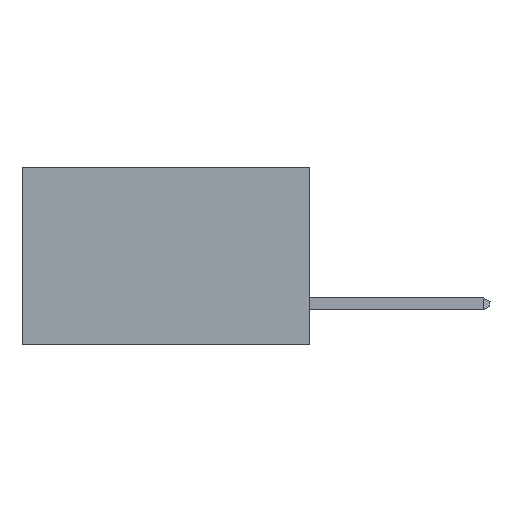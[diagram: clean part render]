
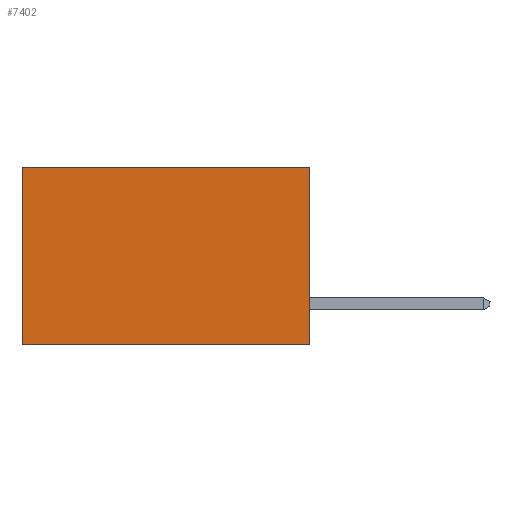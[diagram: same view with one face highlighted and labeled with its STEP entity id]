
A CAD part, left-side view. The second image highlights one B-rep face of the part: STEP entity #7402.
In plain terms, the highlighted planar face has unit normal (-1, 0, 0).
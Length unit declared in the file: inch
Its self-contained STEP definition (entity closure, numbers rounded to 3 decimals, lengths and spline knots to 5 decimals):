
#2269 = VECTOR ( 'NONE', #13233, 39.37008 ) ;
#2680 = LINE ( 'NONE', #18093, #2269 ) ;
#3606 = ORIENTED_EDGE ( 'NONE', *, *, #5074, .F. ) ;
#5074 = EDGE_CURVE ( 'NONE', #19705, #22092, #2680, .T. ) ;
#6584 = EDGE_CURVE ( 'NONE', #19705, #29613, #7545, .T. ) ;
#7337 = DIRECTION ( 'NONE',  ( 0., 0., -1. ) ) ;
#7402 = ADVANCED_FACE ( 'NONE', ( #11373 ), #29030, .F. ) ;
#7545 = LINE ( 'NONE', #10958, #28023 ) ;
#8301 = ORIENTED_EDGE ( 'NONE', *, *, #22850, .T. ) ;
#8864 = LINE ( 'NONE', #15539, #23919 ) ;
#9128 = ORIENTED_EDGE ( 'NONE', *, *, #9698, .F. ) ;
#9698 = EDGE_CURVE ( 'NONE', #22092, #19386, #8864, .T. ) ;
#10958 = CARTESIAN_POINT ( 'NONE',  ( 0.2875, 0., 0. ) ) ;
#11373 = FACE_OUTER_BOUND ( 'NONE', #11970, .T. ) ;
#11970 = EDGE_LOOP ( 'NONE', ( #8301, #9128, #3606, #17429 ) ) ;
#13233 = DIRECTION ( 'NONE',  ( 0., 0., -1. ) ) ;
#14078 = CARTESIAN_POINT ( 'NONE',  ( 0.2875, 0., -0.37 ) ) ;
#15539 = CARTESIAN_POINT ( 'NONE',  ( 0.2875, 0., -0.37 ) ) ;
#17429 = ORIENTED_EDGE ( 'NONE', *, *, #6584, .T. ) ;
#18093 = CARTESIAN_POINT ( 'NONE',  ( 0.2875, 0., 0. ) ) ;
#19191 = DIRECTION ( 'NONE',  ( 1., 0., 0. ) ) ;
#19386 = VERTEX_POINT ( 'NONE', #30410 ) ;
#19705 = VERTEX_POINT ( 'NONE', #24441 ) ;
#21494 = CARTESIAN_POINT ( 'NONE',  ( 0.2875, 0., 0. ) ) ;
#22092 = VERTEX_POINT ( 'NONE', #14078 ) ;
#22850 = EDGE_CURVE ( 'NONE', #29613, #19386, #27058, .T. ) ;
#22922 = DIRECTION ( 'NONE',  ( 0., 1., 0. ) ) ;
#23388 = DIRECTION ( 'NONE',  ( 0., 1., 0. ) ) ;
#23919 = VECTOR ( 'NONE', #22922, 39.37008 ) ;
#23963 = VECTOR ( 'NONE', #7337, 39.37008 ) ;
#24441 = CARTESIAN_POINT ( 'NONE',  ( 0.2875, 0., 0. ) ) ;
#26117 = AXIS2_PLACEMENT_3D ( 'NONE', #21494, #19191, #26322 ) ;
#26322 = DIRECTION ( 'NONE',  ( 0., 0., -1. ) ) ;
#27058 = LINE ( 'NONE', #31753, #23963 ) ;
#28023 = VECTOR ( 'NONE', #23388, 39.37008 ) ;
#28281 = CARTESIAN_POINT ( 'NONE',  ( 0.2875, 0.6, 0. ) ) ;
#29030 = PLANE ( 'NONE',  #26117 ) ;
#29613 = VERTEX_POINT ( 'NONE', #28281 ) ;
#30410 = CARTESIAN_POINT ( 'NONE',  ( 0.2875, 0.6, -0.37 ) ) ;
#31753 = CARTESIAN_POINT ( 'NONE',  ( 0.2875, 0.6, 0. ) ) ;
